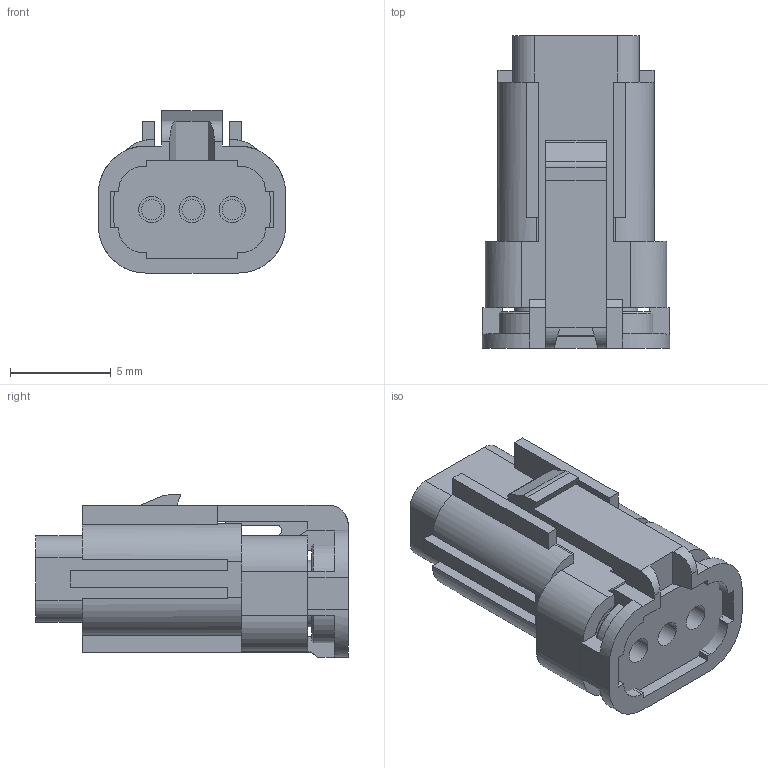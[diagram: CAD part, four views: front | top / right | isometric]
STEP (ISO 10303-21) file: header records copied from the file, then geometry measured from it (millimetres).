
FILE_DESCRIPTION (( 'STEP AP203' ), '1' );
FILE_NAME ('566-003-000-810.STEP', '2021-09-21T18:45:51', ( '' ), ( '' ), 'SwSTEP 2.0', 'SolidWorks 2020', '' );
FILE_SCHEMA (( 'CONFIG_CONTROL_DESIGN' ));
Length unit declared in the file: millimetre
Products named in the file (1): 566-003-000-810
Bounding box: 9.3 x 15.5 x 8.04 mm (x, y, z)
Volume: 554.7 mm3; surface area: 1138.4 mm2
Topology: 2 solids, 2 shells, 406 faces, 1130 edges, 732 vertices
Faces by surface type: plane 305, cylinder 81, torus 16, cone 4
Entity records: 12973 total; most frequent: CARTESIAN_POINT 2275, ORIENTED_EDGE 2260, DIRECTION 2158, EDGE_CURVE 1130, VECTOR 912, LINE 912, VERTEX_POINT 732, AXIS2_PLACEMENT_3D 623
